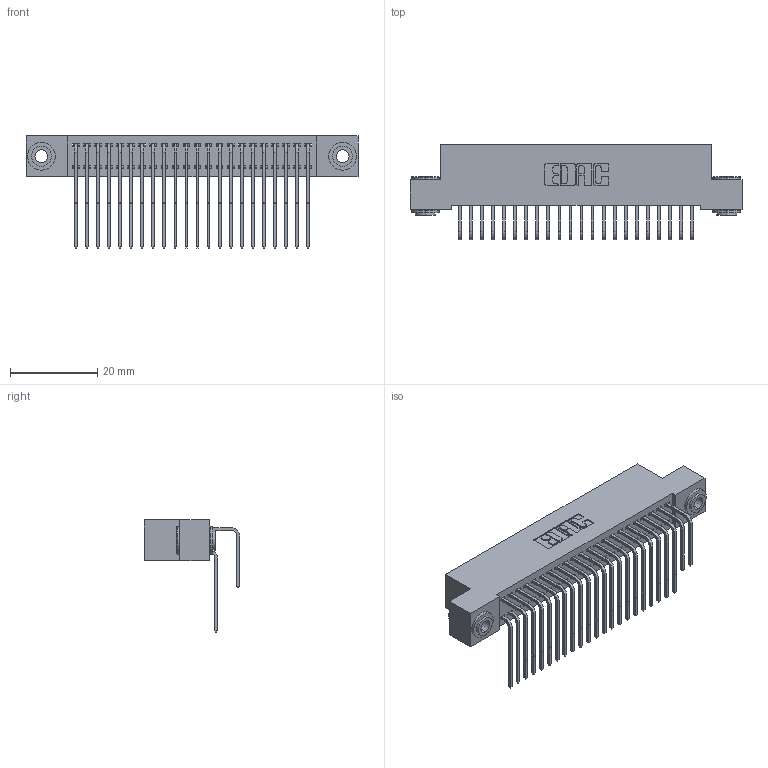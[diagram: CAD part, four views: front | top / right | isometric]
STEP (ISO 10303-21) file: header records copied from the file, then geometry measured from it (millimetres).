
FILE_DESCRIPTION (( 'STEP AP203' ), '1' );
FILE_NAME ('342-044-558-203.STEP', '2019-10-02T19:33:12', ( '' ), ( '' ), 'SwSTEP 2.0', 'SolidWorks 2016', '' );
FILE_SCHEMA (( 'CONFIG_CONTROL_DESIGN' ));
Length unit declared in the file: inch
Products named in the file (5): 342 Part_.156 TH; 345-292-001_558 559 Tail - 1; 345-292-001_558 Tail - 2; 342-250-002_345-250-002-102; 342-044-558-203
Assembly tree (47 placements, depth 2):
  342-044-558-203
    342 Part_.156 TH
    345-292-001_558 559 Tail - 1  x22
    345-292-001_558 Tail - 2  x22
    342-250-002_345-250-002-102  x2
Bounding box: 76.2 x 21.91 x 25.78 mm (x, y, z)
Volume: 7028.5 mm3; surface area: 12310.2 mm2
Topology: 47 solids, 47 shells, 2524 faces, 7459 edges, 4910 vertices
Faces by surface type: plane 1748, cylinder 768, cone 8
Entity records: 19042 total; most frequent: CARTESIAN_POINT 3204, ORIENTED_EDGE 3082, DIRECTION 2787, EDGE_CURVE 1541, LINE 1349, VECTOR 1349, VERTEX_POINT 1022, AXIS2_PLACEMENT_3D 719
